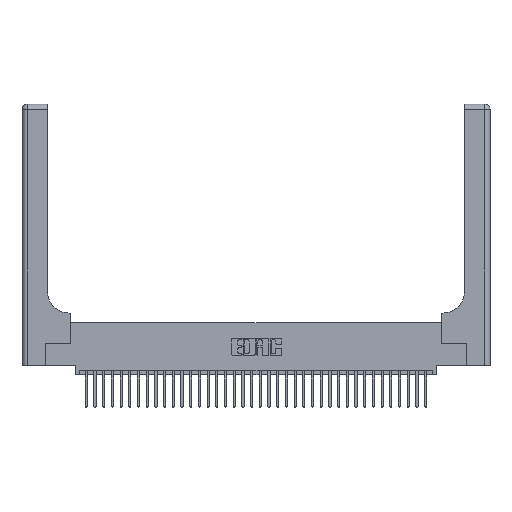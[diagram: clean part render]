
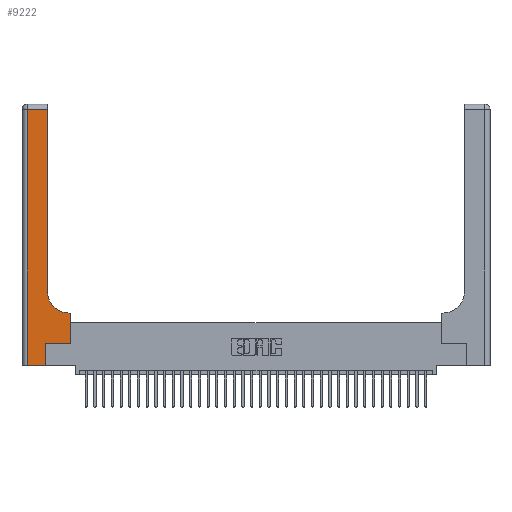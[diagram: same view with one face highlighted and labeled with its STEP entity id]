
A CAD part, top view. The second image highlights one B-rep face of the part: STEP entity #9222.
In plain terms, the highlighted planar face has unit normal (0, 0, 1).
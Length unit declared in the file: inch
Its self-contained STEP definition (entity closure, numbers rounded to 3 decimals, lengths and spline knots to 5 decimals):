
#496 = CARTESIAN_POINT ( 'NONE',  ( 0., 0., 0.37 ) ) ;
#633 = DIRECTION ( 'NONE',  ( -1., 0., 0. ) ) ;
#749 = VECTOR ( 'NONE', #19862, 39.37008 ) ;
#862 = AXIS2_PLACEMENT_3D ( 'NONE', #1611, #21792, #4524 ) ;
#1172 = EDGE_CURVE ( 'NONE', #1366, #25020, #4992, .T. ) ;
#1366 = VERTEX_POINT ( 'NONE', #32768 ) ;
#1611 = CARTESIAN_POINT ( 'NONE',  ( 0.5415, 0.85, 0.37 ) ) ;
#2120 = ORIENTED_EDGE ( 'NONE', *, *, #15791, .T. ) ;
#2229 = EDGE_CURVE ( 'NONE', #30077, #2978, #9400, .T. ) ;
#2562 = CARTESIAN_POINT ( 'NONE',  ( 0., 2.94, 0.37 ) ) ;
#2830 = CARTESIAN_POINT ( 'NONE',  ( 0., 3., 0.37 ) ) ;
#2978 = VERTEX_POINT ( 'NONE', #5074 ) ;
#3430 = DIRECTION ( 'NONE',  ( 1., 0., 0. ) ) ;
#3434 = VECTOR ( 'NONE', #34729, 39.37008 ) ;
#4524 = DIRECTION ( 'NONE',  ( 1., 0., 0. ) ) ;
#4843 = DIRECTION ( 'NONE',  ( 0., -1., 0. ) ) ;
#4992 = LINE ( 'NONE', #496, #23034 ) ;
#5074 = CARTESIAN_POINT ( 'NONE',  ( 0.5585, 0.6, 0.37 ) ) ;
#5741 = DIRECTION ( 'NONE',  ( -1., 0., 0. ) ) ;
#6194 = ORIENTED_EDGE ( 'NONE', *, *, #1172, .T. ) ;
#6368 = EDGE_CURVE ( 'NONE', #36382, #1366, #17691, .T. ) ;
#6462 = CARTESIAN_POINT ( 'NONE',  ( 0.2915, 0.6, 0.37 ) ) ;
#7305 = ORIENTED_EDGE ( 'NONE', *, *, #6368, .T. ) ;
#8178 = CARTESIAN_POINT ( 'NONE',  ( 0.5585, 0.25, 0.37 ) ) ;
#8265 = EDGE_CURVE ( 'NONE', #17846, #36382, #23769, .T. ) ;
#8523 = ORIENTED_EDGE ( 'NONE', *, *, #31574, .T. ) ;
#8687 = ORIENTED_EDGE ( 'NONE', *, *, #8265, .T. ) ;
#9222 = ADVANCED_FACE ( 'NONE', ( #29035 ), #20130, .F. ) ;
#9334 = CARTESIAN_POINT ( 'NONE',  ( 0.269, 0.25, 0.37 ) ) ;
#9400 = LINE ( 'NONE', #8178, #17061 ) ;
#10028 = VECTOR ( 'NONE', #4843, 39.37008 ) ;
#11983 = CARTESIAN_POINT ( 'NONE',  ( 0.2915, 3., 0.37 ) ) ;
#12000 = LINE ( 'NONE', #11983, #3434 ) ;
#12055 = ORIENTED_EDGE ( 'NONE', *, *, #27194, .T. ) ;
#12641 = LINE ( 'NONE', #29863, #34448 ) ;
#13020 = VERTEX_POINT ( 'NONE', #15046 ) ;
#14378 = VECTOR ( 'NONE', #633, 39.37008 ) ;
#14998 = EDGE_LOOP ( 'NONE', ( #12055, #8687, #7305, #6194, #28485, #2120, #24665, #25599, #8523 ) ) ;
#15046 = CARTESIAN_POINT ( 'NONE',  ( 0.269, 0.25, 0.37 ) ) ;
#15791 = EDGE_CURVE ( 'NONE', #13020, #30077, #30737, .T. ) ;
#17061 = VECTOR ( 'NONE', #33702, 39.37008 ) ;
#17691 = LINE ( 'NONE', #27653, #10028 ) ;
#17846 = VERTEX_POINT ( 'NONE', #18751 ) ;
#18470 = DIRECTION ( 'NONE',  ( 0., 1., 0. ) ) ;
#18751 = CARTESIAN_POINT ( 'NONE',  ( 0.2915, 2.94, 0.37 ) ) ;
#19719 = AXIS2_PLACEMENT_3D ( 'NONE', #2830, #23008, #5741 ) ;
#19862 = DIRECTION ( 'NONE',  ( -1., 0., 0. ) ) ;
#20130 = PLANE ( 'NONE',  #19719 ) ;
#21792 = DIRECTION ( 'NONE',  ( 0., 0., -1. ) ) ;
#23008 = DIRECTION ( 'NONE',  ( 0., 0., -1. ) ) ;
#23034 = VECTOR ( 'NONE', #3430, 39.37008 ) ;
#23769 = LINE ( 'NONE', #2562, #749 ) ;
#23815 = CARTESIAN_POINT ( 'NONE',  ( 0.269, 0., 0.37 ) ) ;
#23901 = CARTESIAN_POINT ( 'NONE',  ( 0.06, 2.94, 0.37 ) ) ;
#24665 = ORIENTED_EDGE ( 'NONE', *, *, #2229, .T. ) ;
#25020 = VERTEX_POINT ( 'NONE', #23815 ) ;
#25599 = ORIENTED_EDGE ( 'NONE', *, *, #32458, .T. ) ;
#25838 = CARTESIAN_POINT ( 'NONE',  ( 0.5585, 0.25, 0.37 ) ) ;
#26127 = CARTESIAN_POINT ( 'NONE',  ( 0.5415, 0.6, 0.37 ) ) ;
#26494 = DIRECTION ( 'NONE',  ( 1., 0., 0. ) ) ;
#27194 = EDGE_CURVE ( 'NONE', #36255, #17846, #12000, .T. ) ;
#27653 = CARTESIAN_POINT ( 'NONE',  ( 0.06, 3., 0.37 ) ) ;
#28485 = ORIENTED_EDGE ( 'NONE', *, *, #30377, .T. ) ;
#29035 = FACE_OUTER_BOUND ( 'NONE', #14998, .T. ) ;
#29863 = CARTESIAN_POINT ( 'NONE',  ( 0.269, 0., 0.37 ) ) ;
#30077 = VERTEX_POINT ( 'NONE', #25838 ) ;
#30377 = EDGE_CURVE ( 'NONE', #25020, #13020, #12641, .T. ) ;
#30737 = LINE ( 'NONE', #9334, #36427 ) ;
#31574 = EDGE_CURVE ( 'NONE', #33003, #36255, #32662, .T. ) ;
#32458 = EDGE_CURVE ( 'NONE', #2978, #33003, #33480, .T. ) ;
#32662 = CIRCLE ( 'NONE', #862, 0.25 ) ;
#32768 = CARTESIAN_POINT ( 'NONE',  ( 0.06, 0., 0.37 ) ) ;
#33003 = VERTEX_POINT ( 'NONE', #26127 ) ;
#33480 = LINE ( 'NONE', #6462, #14378 ) ;
#33702 = DIRECTION ( 'NONE',  ( 0., 1., 0. ) ) ;
#34448 = VECTOR ( 'NONE', #18470, 39.37008 ) ;
#34459 = CARTESIAN_POINT ( 'NONE',  ( 0.2915, 0.85, 0.37 ) ) ;
#34729 = DIRECTION ( 'NONE',  ( 0., 1., 0. ) ) ;
#36255 = VERTEX_POINT ( 'NONE', #34459 ) ;
#36382 = VERTEX_POINT ( 'NONE', #23901 ) ;
#36427 = VECTOR ( 'NONE', #26494, 39.37008 ) ;
